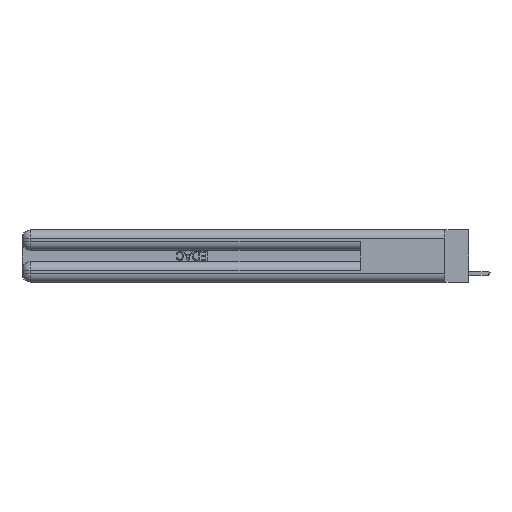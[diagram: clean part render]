
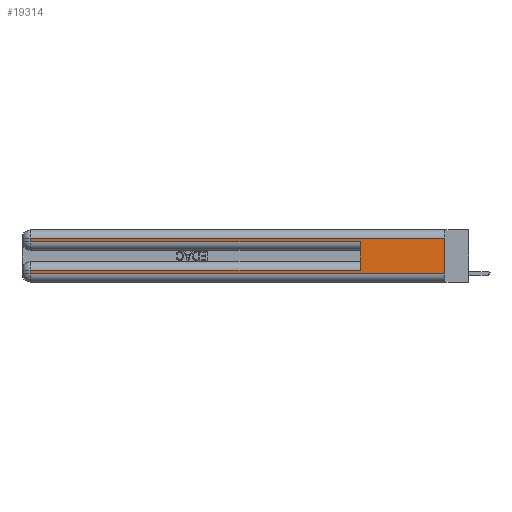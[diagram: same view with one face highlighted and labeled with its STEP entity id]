
A CAD part, left-side view. The second image highlights one B-rep face of the part: STEP entity #19314.
In plain terms, the highlighted planar face has unit normal (-1, 0, 0).
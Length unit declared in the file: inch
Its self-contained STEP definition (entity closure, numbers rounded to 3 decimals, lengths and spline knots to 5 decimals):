
#209 = CARTESIAN_POINT ( 'NONE',  ( 0., 0.6, 0.145 ) ) ;
#791 = VERTEX_POINT ( 'NONE', #7564 ) ;
#892 = EDGE_CURVE ( 'NONE', #10055, #7971, #29736, .T. ) ;
#1458 = ORIENTED_EDGE ( 'NONE', *, *, #892, .T. ) ;
#2739 = CARTESIAN_POINT ( 'NONE',  ( 0., 0., 0.285 ) ) ;
#3374 = EDGE_CURVE ( 'NONE', #25228, #7971, #30522, .T. ) ;
#3902 = DIRECTION ( 'NONE',  ( 0., 1., 0. ) ) ;
#4018 = EDGE_CURVE ( 'NONE', #25228, #4346, #31656, .T. ) ;
#4346 = VERTEX_POINT ( 'NONE', #27446 ) ;
#5414 = CARTESIAN_POINT ( 'NONE',  ( 0., 2.94, 0.285 ) ) ;
#6105 = DIRECTION ( 'NONE',  ( 1., 0., 0. ) ) ;
#6646 = EDGE_LOOP ( 'NONE', ( #12868, #8899, #31723, #25237, #29942, #17906, #10460, #1458 ) ) ;
#6707 = LINE ( 'NONE', #6866, #18070 ) ;
#6866 = CARTESIAN_POINT ( 'NONE',  ( 0., 2.94, 0.37 ) ) ;
#7542 = DIRECTION ( 'NONE',  ( 0., 0., -1. ) ) ;
#7564 = CARTESIAN_POINT ( 'NONE',  ( 0., 2.94, 0.085 ) ) ;
#7971 = VERTEX_POINT ( 'NONE', #23949 ) ;
#8207 = FACE_OUTER_BOUND ( 'NONE', #6646, .T. ) ;
#8899 = ORIENTED_EDGE ( 'NONE', *, *, #4018, .T. ) ;
#10055 = VERTEX_POINT ( 'NONE', #20131 ) ;
#10205 = VERTEX_POINT ( 'NONE', #19454 ) ;
#10460 = ORIENTED_EDGE ( 'NONE', *, *, #32147, .T. ) ;
#11764 = VECTOR ( 'NONE', #25102, 39.37008 ) ;
#12266 = DIRECTION ( 'NONE',  ( 0., 0., -1. ) ) ;
#12304 = EDGE_CURVE ( 'NONE', #15074, #13278, #30856, .T. ) ;
#12868 = ORIENTED_EDGE ( 'NONE', *, *, #3374, .F. ) ;
#13278 = VERTEX_POINT ( 'NONE', #20090 ) ;
#13662 = PLANE ( 'NONE',  #15518 ) ;
#13784 = VECTOR ( 'NONE', #25339, 39.37008 ) ;
#15074 = VERTEX_POINT ( 'NONE', #5414 ) ;
#15518 = AXIS2_PLACEMENT_3D ( 'NONE', #21163, #6105, #25859 ) ;
#17505 = CARTESIAN_POINT ( 'NONE',  ( 0., 2.94, 0.37 ) ) ;
#17599 = DIRECTION ( 'NONE',  ( 0., 0., 1. ) ) ;
#17906 = ORIENTED_EDGE ( 'NONE', *, *, #20180, .T. ) ;
#18070 = VECTOR ( 'NONE', #31988, 39.37008 ) ;
#18074 = VECTOR ( 'NONE', #12266, 39.37008 ) ;
#19137 = VECTOR ( 'NONE', #30208, 39.37008 ) ;
#19314 = ADVANCED_FACE ( 'NONE', ( #8207 ), #13662, .F. ) ;
#19454 = CARTESIAN_POINT ( 'NONE',  ( 0., 0.6, 0.085 ) ) ;
#19968 = CARTESIAN_POINT ( 'NONE',  ( 0., 0., 0.31 ) ) ;
#20090 = CARTESIAN_POINT ( 'NONE',  ( 0., 0.6, 0.285 ) ) ;
#20131 = CARTESIAN_POINT ( 'NONE',  ( 0., 2.94, 0.06 ) ) ;
#20180 = EDGE_CURVE ( 'NONE', #10205, #791, #26474, .T. ) ;
#20744 = VECTOR ( 'NONE', #17599, 39.37008 ) ;
#21163 = CARTESIAN_POINT ( 'NONE',  ( 0., 0., 0.37 ) ) ;
#23346 = EDGE_CURVE ( 'NONE', #4346, #15074, #25839, .T. ) ;
#23894 = VECTOR ( 'NONE', #7542, 39.37008 ) ;
#23949 = CARTESIAN_POINT ( 'NONE',  ( 0., 0., 0.06 ) ) ;
#24242 = LINE ( 'NONE', #209, #20744 ) ;
#24365 = EDGE_CURVE ( 'NONE', #10205, #13278, #24242, .T. ) ;
#25102 = DIRECTION ( 'NONE',  ( 0., 1., 0. ) ) ;
#25228 = VERTEX_POINT ( 'NONE', #28748 ) ;
#25237 = ORIENTED_EDGE ( 'NONE', *, *, #12304, .T. ) ;
#25339 = DIRECTION ( 'NONE',  ( 0., -1., 0. ) ) ;
#25839 = LINE ( 'NONE', #17505, #18074 ) ;
#25859 = DIRECTION ( 'NONE',  ( 0., 0., -1. ) ) ;
#26474 = LINE ( 'NONE', #29288, #29956 ) ;
#27446 = CARTESIAN_POINT ( 'NONE',  ( 0., 2.94, 0.31 ) ) ;
#28748 = CARTESIAN_POINT ( 'NONE',  ( 0., 0., 0.31 ) ) ;
#29288 = CARTESIAN_POINT ( 'NONE',  ( 0., 0., 0.085 ) ) ;
#29736 = LINE ( 'NONE', #30675, #13784 ) ;
#29942 = ORIENTED_EDGE ( 'NONE', *, *, #24365, .F. ) ;
#29956 = VECTOR ( 'NONE', #3902, 39.37008 ) ;
#30208 = DIRECTION ( 'NONE',  ( 0., -1., 0. ) ) ;
#30522 = LINE ( 'NONE', #32014, #23894 ) ;
#30675 = CARTESIAN_POINT ( 'NONE',  ( 0., 0., 0.06 ) ) ;
#30856 = LINE ( 'NONE', #2739, #19137 ) ;
#31656 = LINE ( 'NONE', #19968, #11764 ) ;
#31723 = ORIENTED_EDGE ( 'NONE', *, *, #23346, .T. ) ;
#31988 = DIRECTION ( 'NONE',  ( 0., 0., -1. ) ) ;
#32014 = CARTESIAN_POINT ( 'NONE',  ( 0., 0., 0.37 ) ) ;
#32147 = EDGE_CURVE ( 'NONE', #791, #10055, #6707, .T. ) ;
